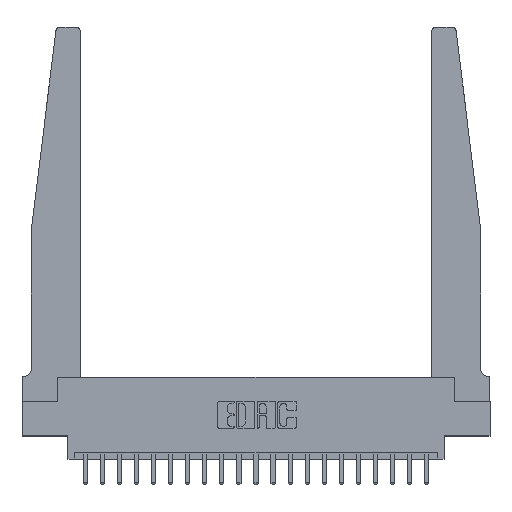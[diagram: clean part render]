
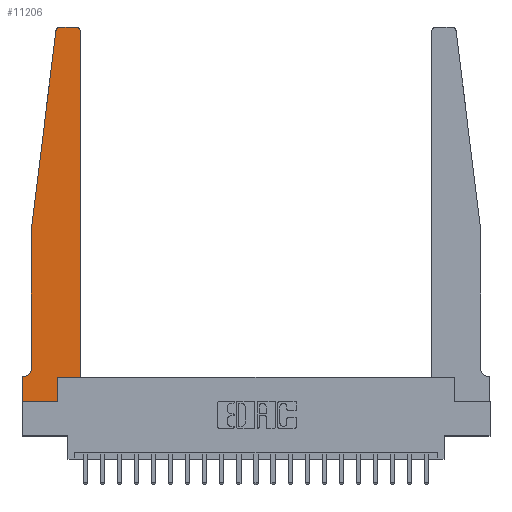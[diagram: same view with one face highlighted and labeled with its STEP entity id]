
A CAD part, top view. The second image highlights one B-rep face of the part: STEP entity #11206.
In plain terms, the highlighted planar face has unit normal (0, 0, 1).
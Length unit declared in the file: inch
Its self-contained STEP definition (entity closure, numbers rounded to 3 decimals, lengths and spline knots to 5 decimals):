
#302 = ORIENTED_EDGE ( 'NONE', *, *, #20254, .T. ) ;
#385 = VERTEX_POINT ( 'NONE', #16538 ) ;
#1447 = CARTESIAN_POINT ( 'NONE',  ( 0.395, 2.75, 0.37 ) ) ;
#2350 = VECTOR ( 'NONE', #19901, 39.37008 ) ;
#2417 = LINE ( 'NONE', #2778, #10901 ) ;
#2635 = EDGE_CURVE ( 'NONE', #10248, #12039, #2417, .T. ) ;
#2723 = DIRECTION ( 'NONE',  ( -1., 0., 0. ) ) ;
#2762 = VERTEX_POINT ( 'NONE', #14690 ) ;
#2778 = CARTESIAN_POINT ( 'NONE',  ( 0.25, 2.75, 0.37 ) ) ;
#2846 = CIRCLE ( 'NONE', #18864, 0.05 ) ;
#3583 = LINE ( 'NONE', #19702, #15208 ) ;
#3889 = LINE ( 'NONE', #9369, #16449 ) ;
#3916 = ORIENTED_EDGE ( 'NONE', *, *, #4672, .T. ) ;
#4067 = ORIENTED_EDGE ( 'NONE', *, *, #20553, .T. ) ;
#4219 = CARTESIAN_POINT ( 'NONE',  ( 0.2605, 0.18, 0.37 ) ) ;
#4656 = ORIENTED_EDGE ( 'NONE', *, *, #2635, .T. ) ;
#4672 = EDGE_CURVE ( 'NONE', #17419, #12803, #20869, .T. ) ;
#5114 = CARTESIAN_POINT ( 'NONE',  ( 0.395, 2.72, 0.37 ) ) ;
#5209 = DIRECTION ( 'NONE',  ( 0., -1., 0. ) ) ;
#6061 = VERTEX_POINT ( 'NONE', #16019 ) ;
#6221 = AXIS2_PLACEMENT_3D ( 'NONE', #17689, #9714, #20921 ) ;
#6440 = CARTESIAN_POINT ( 'NONE',  ( 0.065, 0.2375, 0.37 ) ) ;
#6676 = EDGE_CURVE ( 'NONE', #13437, #17414, #2846, .T. ) ;
#6883 = DIRECTION ( 'NONE',  ( 1., 0., 0. ) ) ;
#6920 = VECTOR ( 'NONE', #19151, 39.37008 ) ;
#7441 = LINE ( 'NONE', #20702, #6920 ) ;
#7669 = DIRECTION ( 'NONE',  ( 0., 0., 1. ) ) ;
#7829 = CARTESIAN_POINT ( 'NONE',  ( 0.015, 0.2375, 0.37 ) ) ;
#8586 = DIRECTION ( 'NONE',  ( -0.122, -0.992, 0. ) ) ;
#9070 = CARTESIAN_POINT ( 'NONE',  ( 0.2605, 0.18, 0.37 ) ) ;
#9219 = ORIENTED_EDGE ( 'NONE', *, *, #10313, .T. ) ;
#9369 = CARTESIAN_POINT ( 'NONE',  ( 0.065, 0.1875, 0.37 ) ) ;
#9423 = DIRECTION ( 'NONE',  ( -1., 0., 0. ) ) ;
#9714 = DIRECTION ( 'NONE',  ( 0., 0., 1. ) ) ;
#10248 = VERTEX_POINT ( 'NONE', #1447 ) ;
#10313 = EDGE_CURVE ( 'NONE', #12214, #385, #20425, .T. ) ;
#10778 = CARTESIAN_POINT ( 'NONE',  ( 0.015, 0.1875, 0.37 ) ) ;
#10846 = AXIS2_PLACEMENT_3D ( 'NONE', #17219, #7669, #18857 ) ;
#10901 = VECTOR ( 'NONE', #2723, 39.37008 ) ;
#10963 = ORIENTED_EDGE ( 'NONE', *, *, #15470, .T. ) ;
#11177 = VECTOR ( 'NONE', #12253, 39.37008 ) ;
#11206 = ADVANCED_FACE ( 'NONE', ( #13344 ), #20855, .T. ) ;
#12039 = VERTEX_POINT ( 'NONE', #16997 ) ;
#12081 = ORIENTED_EDGE ( 'NONE', *, *, #20781, .T. ) ;
#12214 = VERTEX_POINT ( 'NONE', #15814 ) ;
#12253 = DIRECTION ( 'NONE',  ( 0., 1., 0. ) ) ;
#12384 = ORIENTED_EDGE ( 'NONE', *, *, #15099, .T. ) ;
#12715 = ORIENTED_EDGE ( 'NONE', *, *, #16318, .T. ) ;
#12803 = VERTEX_POINT ( 'NONE', #17258 ) ;
#12941 = CIRCLE ( 'NONE', #10846, 0.03 ) ;
#13209 = DIRECTION ( 'NONE',  ( 1., 0., 0. ) ) ;
#13338 = CIRCLE ( 'NONE', #18925, 0.03 ) ;
#13344 = FACE_OUTER_BOUND ( 'NONE', #17276, .T. ) ;
#13373 = CARTESIAN_POINT ( 'NONE',  ( 0.065, 1.25, 0.37 ) ) ;
#13437 = VERTEX_POINT ( 'NONE', #6440 ) ;
#14452 = VECTOR ( 'NONE', #21213, 39.37008 ) ;
#14504 = ORIENTED_EDGE ( 'NONE', *, *, #14719, .T. ) ;
#14690 = CARTESIAN_POINT ( 'NONE',  ( 0.425, 2.72, 0.37 ) ) ;
#14719 = EDGE_CURVE ( 'NONE', #12039, #12214, #12941, .T. ) ;
#14759 = CARTESIAN_POINT ( 'NONE',  ( 0.425, 0.18, 0.37 ) ) ;
#14768 = CARTESIAN_POINT ( 'NONE',  ( 0.425, 0.18, 0.37 ) ) ;
#15099 = EDGE_CURVE ( 'NONE', #12803, #2762, #19206, .T. ) ;
#15208 = VECTOR ( 'NONE', #5209, 39.37008 ) ;
#15470 = EDGE_CURVE ( 'NONE', #385, #13437, #7441, .T. ) ;
#15598 = LINE ( 'NONE', #18292, #2350 ) ;
#15814 = CARTESIAN_POINT ( 'NONE',  ( 0.24675, 2.72367, 0.37 ) ) ;
#16019 = CARTESIAN_POINT ( 'NONE',  ( 0., 0.1875, 0.37 ) ) ;
#16206 = EDGE_CURVE ( 'NONE', #2762, #10248, #13338, .T. ) ;
#16318 = EDGE_CURVE ( 'NONE', #18197, #18413, #15598, .T. ) ;
#16444 = DIRECTION ( 'NONE',  ( 0., 0., 1. ) ) ;
#16449 = VECTOR ( 'NONE', #17401, 39.37008 ) ;
#16538 = CARTESIAN_POINT ( 'NONE',  ( 0.065, 1.25, 0.37 ) ) ;
#16584 = VECTOR ( 'NONE', #13209, 39.37008 ) ;
#16636 = VECTOR ( 'NONE', #8586, 39.37008 ) ;
#16997 = CARTESIAN_POINT ( 'NONE',  ( 0.27653, 2.75, 0.37 ) ) ;
#17219 = CARTESIAN_POINT ( 'NONE',  ( 0.27653, 2.72, 0.37 ) ) ;
#17258 = CARTESIAN_POINT ( 'NONE',  ( 0.425, 0.18, 0.37 ) ) ;
#17276 = EDGE_LOOP ( 'NONE', ( #4656, #14504, #9219, #10963, #17651, #302, #4067, #12715, #12081, #3916, #12384, #19786 ) ) ;
#17401 = DIRECTION ( 'NONE',  ( -1., 0., 0. ) ) ;
#17414 = VERTEX_POINT ( 'NONE', #10778 ) ;
#17419 = VERTEX_POINT ( 'NONE', #4219 ) ;
#17651 = ORIENTED_EDGE ( 'NONE', *, *, #6676, .T. ) ;
#17678 = CARTESIAN_POINT ( 'NONE',  ( 0., 0., 0.37 ) ) ;
#17689 = CARTESIAN_POINT ( 'NONE',  ( 0., 0.1875, 0.37 ) ) ;
#18197 = VERTEX_POINT ( 'NONE', #17678 ) ;
#18292 = CARTESIAN_POINT ( 'NONE',  ( 0., 0., 0.37 ) ) ;
#18413 = VERTEX_POINT ( 'NONE', #19911 ) ;
#18857 = DIRECTION ( 'NONE',  ( 1., 0., 0. ) ) ;
#18864 = AXIS2_PLACEMENT_3D ( 'NONE', #7829, #19004, #9423 ) ;
#18925 = AXIS2_PLACEMENT_3D ( 'NONE', #5114, #16444, #6883 ) ;
#19004 = DIRECTION ( 'NONE',  ( 0., 0., -1. ) ) ;
#19151 = DIRECTION ( 'NONE',  ( 0., -1., 0. ) ) ;
#19206 = LINE ( 'NONE', #14759, #14452 ) ;
#19702 = CARTESIAN_POINT ( 'NONE',  ( 0., 0., 0.37 ) ) ;
#19705 = LINE ( 'NONE', #9070, #11177 ) ;
#19786 = ORIENTED_EDGE ( 'NONE', *, *, #16206, .T. ) ;
#19901 = DIRECTION ( 'NONE',  ( 1., 0., 0. ) ) ;
#19911 = CARTESIAN_POINT ( 'NONE',  ( 0.2605, 0., 0.37 ) ) ;
#20254 = EDGE_CURVE ( 'NONE', #17414, #6061, #3889, .T. ) ;
#20425 = LINE ( 'NONE', #13373, #16636 ) ;
#20553 = EDGE_CURVE ( 'NONE', #6061, #18197, #3583, .T. ) ;
#20702 = CARTESIAN_POINT ( 'NONE',  ( 0.065, 1.25, 0.37 ) ) ;
#20781 = EDGE_CURVE ( 'NONE', #18413, #17419, #19705, .T. ) ;
#20855 = PLANE ( 'NONE',  #6221 ) ;
#20869 = LINE ( 'NONE', #14768, #16584 ) ;
#20921 = DIRECTION ( 'NONE',  ( 1., 0., 0. ) ) ;
#21213 = DIRECTION ( 'NONE',  ( 0., 1., 0. ) ) ;
